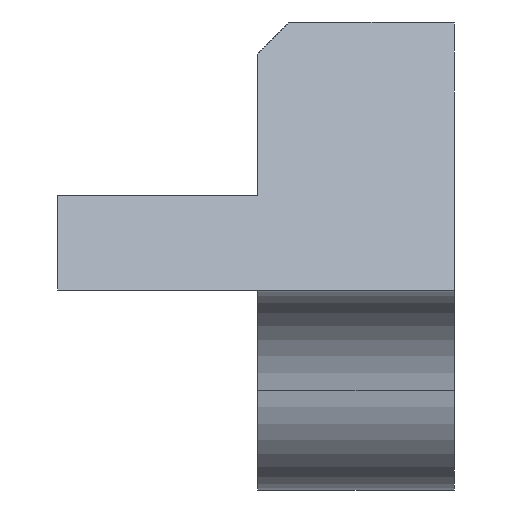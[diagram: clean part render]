
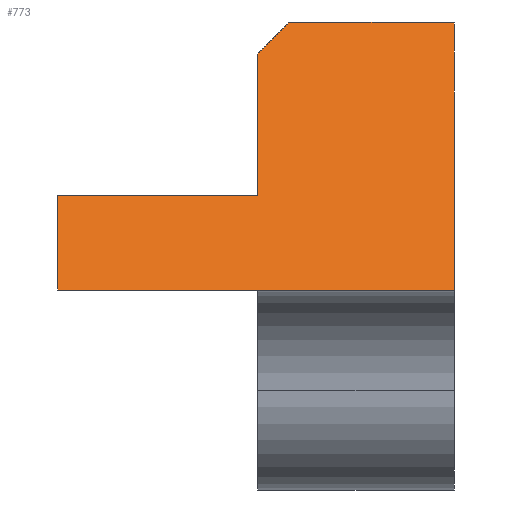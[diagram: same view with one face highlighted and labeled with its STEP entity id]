
A CAD part, left-side view. The second image highlights one B-rep face of the part: STEP entity #773.
In plain terms, the highlighted planar face has unit normal (-0.707, 0, 0.707).
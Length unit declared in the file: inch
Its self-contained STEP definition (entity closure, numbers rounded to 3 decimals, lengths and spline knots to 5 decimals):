
#7 = CARTESIAN_POINT ( 'NONE',  ( -1.087, 2.03695, 0.113 ) ) ;
#24 = CARTESIAN_POINT ( 'NONE',  ( -1.1475, -0.123, 0.0525 ) ) ;
#26 = LINE ( 'NONE', #424, #323 ) ;
#30 = VERTEX_POINT ( 'NONE', #759 ) ;
#48 = AXIS2_PLACEMENT_3D ( 'NONE', #7, #554, #184 ) ;
#69 = VERTEX_POINT ( 'NONE', #568 ) ;
#87 = LINE ( 'NONE', #24, #553 ) ;
#100 = LINE ( 'NONE', #699, #577 ) ;
#103 = VERTEX_POINT ( 'NONE', #458 ) ;
#158 = VECTOR ( 'NONE', #753, 39.37008 ) ;
#184 = DIRECTION ( 'NONE',  ( 0.707, 0., 0.707 ) ) ;
#193 = ORIENTED_EDGE ( 'NONE', *, *, #616, .T. ) ;
#220 = CARTESIAN_POINT ( 'NONE',  ( -1.375, 0.123, -0.175 ) ) ;
#245 = PLANE ( 'NONE',  #48 ) ;
#282 = DIRECTION ( 'NONE',  ( 0., -1., 0. ) ) ;
#302 = FACE_OUTER_BOUND ( 'NONE', #706, .T. ) ;
#307 = CARTESIAN_POINT ( 'NONE',  ( -1.25689, 0.373, -0.05689 ) ) ;
#308 = CARTESIAN_POINT ( 'NONE',  ( -1.25689, 0.68633, -0.05689 ) ) ;
#319 = DIRECTION ( 'NONE',  ( 0.577, -0.577, 0.577 ) ) ;
#323 = VECTOR ( 'NONE', #486, 39.37008 ) ;
#330 = VERTEX_POINT ( 'NONE', #545 ) ;
#352 = ORIENTED_EDGE ( 'NONE', *, *, #597, .F. ) ;
#367 = CARTESIAN_POINT ( 'NONE',  ( -1.375, 0.373, -0.175 ) ) ;
#424 = CARTESIAN_POINT ( 'NONE',  ( -0.6, 0.373, 0.6 ) ) ;
#428 = VECTOR ( 'NONE', #615, 39.37008 ) ;
#437 = ORIENTED_EDGE ( 'NONE', *, *, #776, .F. ) ;
#458 = CARTESIAN_POINT ( 'NONE',  ( -1.04, -0.123, 0.16 ) ) ;
#479 = VERTEX_POINT ( 'NONE', #367 ) ;
#486 = DIRECTION ( 'NONE',  ( 0.707, 0., 0.707 ) ) ;
#514 = ORIENTED_EDGE ( 'NONE', *, *, #741, .F. ) ;
#523 = DIRECTION ( 'NONE',  ( 0., -1., 0. ) ) ;
#545 = CARTESIAN_POINT ( 'NONE',  ( -1.25689, 0.123, -0.05689 ) ) ;
#553 = VECTOR ( 'NONE', #769, 39.37008 ) ;
#554 = DIRECTION ( 'NONE',  ( -0.707, 0., 0.707 ) ) ;
#557 = CARTESIAN_POINT ( 'NONE',  ( -1.0675, 0.123, 0.1325 ) ) ;
#560 = ORIENTED_EDGE ( 'NONE', *, *, #792, .T. ) ;
#568 = CARTESIAN_POINT ( 'NONE',  ( -1.08, 0.123, 0.12 ) ) ;
#569 = VECTOR ( 'NONE', #282, 39.37008 ) ;
#577 = VECTOR ( 'NONE', #319, 39.37008 ) ;
#590 = CARTESIAN_POINT ( 'NONE',  ( -1.04, 0.083, 0.16 ) ) ;
#597 = EDGE_CURVE ( 'NONE', #69, #669, #100, .T. ) ;
#602 = VECTOR ( 'NONE', #523, 39.37008 ) ;
#612 = LINE ( 'NONE', #308, #158 ) ;
#615 = DIRECTION ( 'NONE',  ( -0.707, 0., -0.707 ) ) ;
#616 = EDGE_CURVE ( 'NONE', #30, #103, #87, .T. ) ;
#636 = ORIENTED_EDGE ( 'NONE', *, *, #686, .T. ) ;
#646 = EDGE_CURVE ( 'NONE', #669, #103, #786, .T. ) ;
#669 = VERTEX_POINT ( 'NONE', #590 ) ;
#686 = EDGE_CURVE ( 'NONE', #479, #30, #738, .T. ) ;
#698 = ORIENTED_EDGE ( 'NONE', *, *, #646, .F. ) ;
#699 = CARTESIAN_POINT ( 'NONE',  ( -1.08233, 0.12533, 0.11767 ) ) ;
#706 = EDGE_LOOP ( 'NONE', ( #636, #193, #698, #352, #560, #437, #514 ) ) ;
#738 = LINE ( 'NONE', #220, #569 ) ;
#741 = EDGE_CURVE ( 'NONE', #479, #771, #26, .T. ) ;
#753 = DIRECTION ( 'NONE',  ( 0., -1., 0. ) ) ;
#759 = CARTESIAN_POINT ( 'NONE',  ( -1.375, -0.123, -0.175 ) ) ;
#769 = DIRECTION ( 'NONE',  ( 0.707, 0., 0.707 ) ) ;
#771 = VERTEX_POINT ( 'NONE', #307 ) ;
#773 = ADVANCED_FACE ( 'NONE', ( #302 ), #245, .T. ) ;
#775 = LINE ( 'NONE', #557, #428 ) ;
#776 = EDGE_CURVE ( 'NONE', #771, #330, #612, .T. ) ;
#786 = LINE ( 'NONE', #790, #602 ) ;
#790 = CARTESIAN_POINT ( 'NONE',  ( -1.04, -0.123, 0.16 ) ) ;
#792 = EDGE_CURVE ( 'NONE', #69, #330, #775, .T. ) ;
